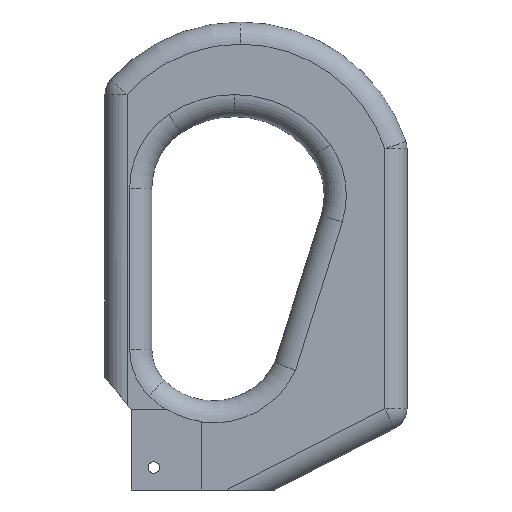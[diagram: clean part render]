
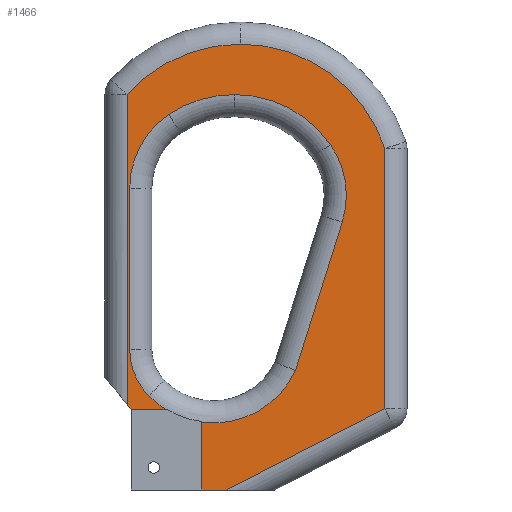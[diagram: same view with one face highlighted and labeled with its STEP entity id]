
A CAD part, left-side view. The second image highlights one B-rep face of the part: STEP entity #1466.
In plain terms, the highlighted planar face has unit normal (-1, 0, 0).
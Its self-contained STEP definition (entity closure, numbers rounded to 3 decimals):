
#19 = AXIS2_PLACEMENT_3D ( 'NONE', #881, #895, #908 ) ;
#24 = AXIS2_PLACEMENT_3D ( 'NONE', #843, #858, #856 ) ;
#28 = AXIS2_PLACEMENT_3D ( 'NONE', #877, #870, #879 ) ;
#30 = VECTOR ( 'NONE', #824, 1000. ) ;
#33 = AXIS2_PLACEMENT_3D ( 'NONE', #891, #892, #885 ) ;
#40 = VECTOR ( 'NONE', #900, 1000. ) ;
#219 = ORIENTED_EDGE ( 'NONE', *, *, #1413, .F. ) ;
#222 = ORIENTED_EDGE ( 'NONE', *, *, #1398, .T. ) ;
#243 = ORIENTED_EDGE ( 'NONE', *, *, #1442, .T. ) ;
#244 = ORIENTED_EDGE ( 'NONE', *, *, #1654, .T. ) ;
#246 = ORIENTED_EDGE ( 'NONE', *, *, #1419, .T. ) ;
#249 = ORIENTED_EDGE ( 'NONE', *, *, #1434, .T. ) ;
#251 = ORIENTED_EDGE ( 'NONE', *, *, #1368, .F. ) ;
#253 = ORIENTED_EDGE ( 'NONE', *, *, #1428, .T. ) ;
#254 = ORIENTED_EDGE ( 'NONE', *, *, #1350, .T. ) ;
#259 = ORIENTED_EDGE ( 'NONE', *, *, #1445, .T. ) ;
#262 = ORIENTED_EDGE ( 'NONE', *, *, #1430, .T. ) ;
#263 = ORIENTED_EDGE ( 'NONE', *, *, #1400, .F. ) ;
#264 = ORIENTED_EDGE ( 'NONE', *, *, #1444, .T. ) ;
#265 = ORIENTED_EDGE ( 'NONE', *, *, #1404, .F. ) ;
#266 = ORIENTED_EDGE ( 'NONE', *, *, #1429, .T. ) ;
#267 = ORIENTED_EDGE ( 'NONE', *, *, #1431, .T. ) ;
#277 = ORIENTED_EDGE ( 'NONE', *, *, #1447, .T. ) ;
#278 = ORIENTED_EDGE ( 'NONE', *, *, #1456, .T. ) ;
#283 = EDGE_LOOP ( 'NONE', ( #244, #222, #246, #219, #263, #243, #259, #266, #249, #262, #254, #277, #278, #253, #265, #251, #267, #264 ) ) ;
#345 = VERTEX_POINT ( 'NONE', #455 ) ;
#359 = VERTEX_POINT ( 'NONE', #446 ) ;
#360 = VERTEX_POINT ( 'NONE', #453 ) ;
#364 = VERTEX_POINT ( 'NONE', #460 ) ;
#378 = VERTEX_POINT ( 'NONE', #502 ) ;
#383 = VERTEX_POINT ( 'NONE', #485 ) ;
#388 = VERTEX_POINT ( 'NONE', #476 ) ;
#393 = VERTEX_POINT ( 'NONE', #486 ) ;
#400 = VERTEX_POINT ( 'NONE', #483 ) ;
#408 = VERTEX_POINT ( 'NONE', #521 ) ;
#411 = VERTEX_POINT ( 'NONE', #515 ) ;
#412 = VERTEX_POINT ( 'NONE', #522 ) ;
#417 = VERTEX_POINT ( 'NONE', #536 ) ;
#419 = VERTEX_POINT ( 'NONE', #525 ) ;
#421 = VERTEX_POINT ( 'NONE', #526 ) ;
#427 = VERTEX_POINT ( 'NONE', #512 ) ;
#428 = VERTEX_POINT ( 'NONE', #532 ) ;
#437 = VERTEX_POINT ( 'NONE', #510 ) ;
#446 = CARTESIAN_POINT ( 'NONE',  ( -11.118, -58.09, 139.346 ) ) ;
#453 = CARTESIAN_POINT ( 'NONE',  ( -11.118, -82.67, 137.583 ) ) ;
#455 = CARTESIAN_POINT ( 'NONE',  ( -11.118, -14.754, 161.929 ) ) ;
#460 = CARTESIAN_POINT ( 'NONE',  ( -11.118, -17.428, 184.666 ) ) ;
#476 = CARTESIAN_POINT ( 'NONE',  ( -11.118, 31.75, 19.685 ) ) ;
#483 = CARTESIAN_POINT ( 'NONE',  ( -11.118, 0., -16.51 ) ) ;
#485 = CARTESIAN_POINT ( 'NONE',  ( -11.118, 0., 14.067 ) ) ;
#486 = CARTESIAN_POINT ( 'NONE',  ( -11.118, 33.61, 21.991 ) ) ;
#502 = CARTESIAN_POINT ( 'NONE',  ( -11.118, -11.053, -16.51 ) ) ;
#510 = CARTESIAN_POINT ( 'NONE',  ( -11.118, 23.877, 25.972 ) ) ;
#512 = CARTESIAN_POINT ( 'NONE',  ( -11.118, 33.61, 161.974 ) ) ;
#515 = CARTESIAN_POINT ( 'NONE',  ( -11.118, 14.84, 152.871 ) ) ;
#521 = CARTESIAN_POINT ( 'NONE',  ( -11.118, 15.964, 19.685 ) ) ;
#522 = CARTESIAN_POINT ( 'NONE',  ( -11.118, -82.67, 20.162 ) ) ;
#525 = CARTESIAN_POINT ( 'NONE',  ( -11.118, 32.451, 119.724 ) ) ;
#526 = CARTESIAN_POINT ( 'NONE',  ( -11.118, -42.325, 37.432 ) ) ;
#532 = CARTESIAN_POINT ( 'NONE',  ( -11.118, 32.451, 46.97 ) ) ;
#536 = CARTESIAN_POINT ( 'NONE',  ( -11.118, -63.451, 104.397 ) ) ;
#573 = DIRECTION ( 'NONE',  ( 1., 0., 0. ) ) ;
#574 = DIRECTION ( 'NONE',  ( 0., 0., 1. ) ) ;
#597 = CARTESIAN_POINT ( 'NONE',  ( -11.118, -14.754, 109.057 ) ) ;
#645 = CARTESIAN_POINT ( 'NONE',  ( -11.118, 0., -16.51 ) ) ;
#658 = LINE ( 'NONE', #645, #1305 ) ;
#662 = DIRECTION ( 'NONE',  ( 0., 1., 0. ) ) ;
#717 = CARTESIAN_POINT ( 'NONE',  ( -11.118, -17.428, 115.922 ) ) ;
#729 = LINE ( 'NONE', #752, #2026 ) ;
#736 = DIRECTION ( 'NONE',  ( -1., 0., 0. ) ) ;
#740 = DIRECTION ( 'NONE',  ( 0., 0., 1. ) ) ;
#742 = DIRECTION ( 'NONE',  ( 0., 1., 0. ) ) ;
#752 = CARTESIAN_POINT ( 'NONE',  ( -11.118, 31.75, 19.685 ) ) ;
#764 = DIRECTION ( 'NONE',  ( 0., 0., 1. ) ) ;
#766 = LINE ( 'NONE', #785, #2000 ) ;
#779 = LINE ( 'NONE', #798, #2006 ) ;
#785 = CARTESIAN_POINT ( 'NONE',  ( -11.118, 0., 19.685 ) ) ;
#794 = DIRECTION ( 'NONE',  ( 0., 0.628, 0.778 ) ) ;
#797 = DIRECTION ( 'NONE',  ( 0., 0., -1. ) ) ;
#798 = CARTESIAN_POINT ( 'NONE',  ( -11.118, 43.61, 34.386 ) ) ;
#813 = LINE ( 'NONE', #816, #2007 ) ;
#816 = CARTESIAN_POINT ( 'NONE',  ( -11.118, 33.61, 115.922 ) ) ;
#822 = CARTESIAN_POINT ( 'NONE',  ( -11.118, -5.271, 54.537 ) ) ;
#823 = DIRECTION ( 'NONE',  ( 1., 0., 0. ) ) ;
#824 = DIRECTION ( 'NONE',  ( 0., -0.89, 0.456 ) ) ;
#825 = DIRECTION ( 'NONE',  ( 0., 0., 1. ) ) ;
#826 = DIRECTION ( 'NONE',  ( 0., 0., 1. ) ) ;
#829 = CARTESIAN_POINT ( 'NONE',  ( -11.118, -69.83, 13.588 ) ) ;
#831 = LINE ( 'NONE', #836, #2021 ) ;
#833 = DIRECTION ( 'NONE',  ( 0., 0., 1. ) ) ;
#836 = CARTESIAN_POINT ( 'NONE',  ( -11.118, 32.451, 119.724 ) ) ;
#837 = LINE ( 'NONE', #829, #30 ) ;
#843 = CARTESIAN_POINT ( 'NONE',  ( -11.118, -7.549, 119.724 ) ) ;
#846 = CARTESIAN_POINT ( 'NONE',  ( -11.118, -14.754, 109.057 ) ) ;
#850 = DIRECTION ( 'NONE',  ( 1., 0., 0. ) ) ;
#854 = LINE ( 'NONE', #855, #40 ) ;
#855 = CARTESIAN_POINT ( 'NONE',  ( -11.118, -82.67, 115.922 ) ) ;
#856 = DIRECTION ( 'NONE',  ( 0., 0., 1. ) ) ;
#858 = DIRECTION ( 'NONE',  ( 1., 0., 0. ) ) ;
#870 = DIRECTION ( 'NONE',  ( 1., 0., 0. ) ) ;
#877 = CARTESIAN_POINT ( 'NONE',  ( -11.118, -5.271, 54.537 ) ) ;
#879 = DIRECTION ( 'NONE',  ( 0., 0., 1. ) ) ;
#881 = CARTESIAN_POINT ( 'NONE',  ( -11.118, 2.451, 46.97 ) ) ;
#885 = DIRECTION ( 'NONE',  ( 0., 0., 1. ) ) ;
#891 = CARTESIAN_POINT ( 'NONE',  ( -11.118, -25.305, 116.431 ) ) ;
#892 = DIRECTION ( 'NONE',  ( 1., 0., 0. ) ) ;
#895 = DIRECTION ( 'NONE',  ( 1., 0., 0. ) ) ;
#900 = DIRECTION ( 'NONE',  ( 0., 0., 1. ) ) ;
#908 = DIRECTION ( 'NONE',  ( 0., 0., 1. ) ) ;
#931 = DIRECTION ( 'NONE',  ( 0., 0.301, -0.954 ) ) ;
#943 = LINE ( 'NONE', #945, #1673 ) ;
#945 = CARTESIAN_POINT ( 'NONE',  ( -11.118, -42.53, 38.08 ) ) ;
#955 = DIRECTION ( 'NONE',  ( 0., 0., 1. ) ) ;
#958 = CARTESIAN_POINT ( 'NONE',  ( -11.118, -17.428, 115.922 ) ) ;
#963 = PLANE ( 'NONE',  #1704 ) ;
#964 = DIRECTION ( 'NONE',  ( -1., 0., 0. ) ) ;
#1270 = DIRECTION ( 'NONE',  ( -1., 0., 0. ) ) ;
#1287 = CARTESIAN_POINT ( 'NONE',  ( -11.118, -17.428, 115.922 ) ) ;
#1288 = DIRECTION ( 'NONE',  ( 0., 0., 1. ) ) ;
#1305 = VECTOR ( 'NONE', #662, 1000. ) ;
#1315 = AXIS2_PLACEMENT_3D ( 'NONE', #597, #573, #574 ) ;
#1350 = EDGE_CURVE ( 'NONE', #345, #359, #1504, .T. ) ;
#1368 = EDGE_CURVE ( 'NONE', #378, #400, #658, .T. ) ;
#1398 = EDGE_CURVE ( 'NONE', #364, #427, #1528, .T. ) ;
#1400 = EDGE_CURVE ( 'NONE', #408, #388, #729, .T. ) ;
#1404 = EDGE_CURVE ( 'NONE', #400, #383, #766, .T. ) ;
#1413 = EDGE_CURVE ( 'NONE', #388, #393, #779, .T. ) ;
#1419 = EDGE_CURVE ( 'NONE', #427, #393, #813, .T. ) ;
#1428 = EDGE_CURVE ( 'NONE', #421, #383, #1522, .T. ) ;
#1429 = EDGE_CURVE ( 'NONE', #428, #419, #831, .T. ) ;
#1430 = EDGE_CURVE ( 'NONE', #411, #345, #1523, .T. ) ;
#1431 = EDGE_CURVE ( 'NONE', #378, #412, #837, .T. ) ;
#1434 = EDGE_CURVE ( 'NONE', #419, #411, #1539, .T. ) ;
#1442 = EDGE_CURVE ( 'NONE', #408, #437, #1530, .T. ) ;
#1444 = EDGE_CURVE ( 'NONE', #412, #360, #854, .T. ) ;
#1445 = EDGE_CURVE ( 'NONE', #437, #428, #1525, .T. ) ;
#1447 = EDGE_CURVE ( 'NONE', #359, #417, #1540, .T. ) ;
#1456 = EDGE_CURVE ( 'NONE', #417, #421, #943, .T. ) ;
#1466 = ADVANCED_FACE ( 'NONE', ( #1702 ), #963, .T. ) ;
#1504 = CIRCLE ( 'NONE', #1315, 52.872 ) ;
#1522 = CIRCLE ( 'NONE', #1998, 40.812 ) ;
#1523 = CIRCLE ( 'NONE', #2020, 52.872 ) ;
#1525 = CIRCLE ( 'NONE', #19, 30. ) ;
#1528 = CIRCLE ( 'NONE', #2033, 68.744 ) ;
#1530 = CIRCLE ( 'NONE', #28, 40.812 ) ;
#1539 = CIRCLE ( 'NONE', #24, 40. ) ;
#1540 = CIRCLE ( 'NONE', #33, 40. ) ;
#1582 = CIRCLE ( 'NONE', #1716, 68.744 ) ;
#1654 = EDGE_CURVE ( 'NONE', #360, #364, #1582, .T. ) ;
#1673 = VECTOR ( 'NONE', #931, 1000. ) ;
#1702 = FACE_OUTER_BOUND ( 'NONE', #283, .T. ) ;
#1704 = AXIS2_PLACEMENT_3D ( 'NONE', #958, #964, #955 ) ;
#1716 = AXIS2_PLACEMENT_3D ( 'NONE', #1287, #1270, #1288 ) ;
#1998 = AXIS2_PLACEMENT_3D ( 'NONE', #822, #823, #826 ) ;
#2000 = VECTOR ( 'NONE', #764, 1000. ) ;
#2006 = VECTOR ( 'NONE', #794, 1000. ) ;
#2007 = VECTOR ( 'NONE', #797, 1000. ) ;
#2020 = AXIS2_PLACEMENT_3D ( 'NONE', #846, #850, #825 ) ;
#2021 = VECTOR ( 'NONE', #833, 1000. ) ;
#2026 = VECTOR ( 'NONE', #742, 1000. ) ;
#2033 = AXIS2_PLACEMENT_3D ( 'NONE', #717, #736, #740 ) ;
